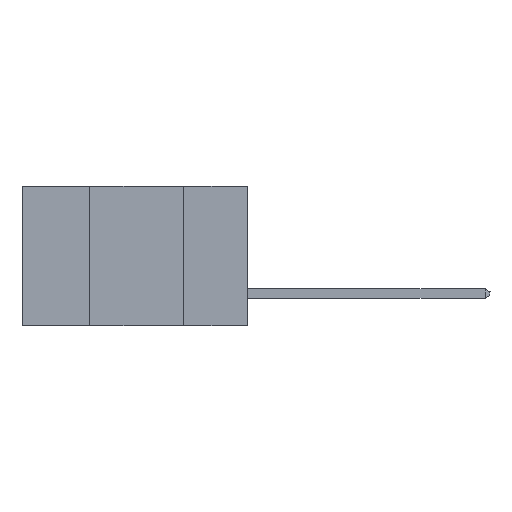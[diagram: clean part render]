
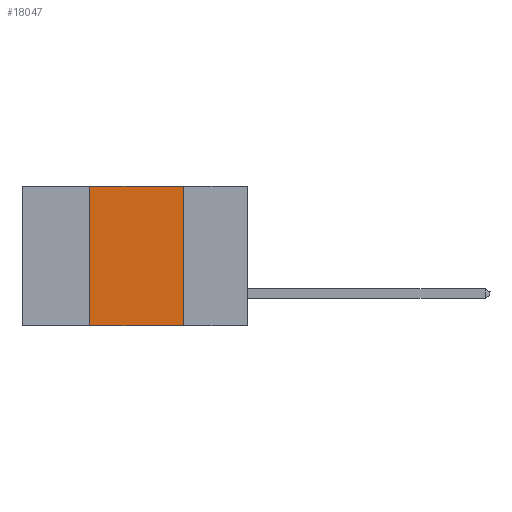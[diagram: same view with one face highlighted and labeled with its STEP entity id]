
A CAD part, left-side view. The second image highlights one B-rep face of the part: STEP entity #18047.
In plain terms, the highlighted planar face has unit normal (-1, 0, 0).
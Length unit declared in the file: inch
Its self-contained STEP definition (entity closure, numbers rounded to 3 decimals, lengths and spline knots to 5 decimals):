
#502 = LINE ( 'NONE', #14498, #7834 ) ;
#1542 = VECTOR ( 'NONE', #5085, 39.37008 ) ;
#1712 = VERTEX_POINT ( 'NONE', #15161 ) ;
#2251 = ORIENTED_EDGE ( 'NONE', *, *, #16528, .F. ) ;
#2305 = DIRECTION ( 'NONE',  ( 0., -1., 0. ) ) ;
#2497 = AXIS2_PLACEMENT_3D ( 'NONE', #5988, #2922, #11907 ) ;
#2922 = DIRECTION ( 'NONE',  ( 1., 0., 0. ) ) ;
#3722 = VERTEX_POINT ( 'NONE', #14908 ) ;
#5085 = DIRECTION ( 'NONE',  ( 0., 0., 1. ) ) ;
#5988 = CARTESIAN_POINT ( 'NONE',  ( 0., 0.6, 0. ) ) ;
#6765 = LINE ( 'NONE', #15477, #15172 ) ;
#7340 = PLANE ( 'NONE',  #2497 ) ;
#7834 = VECTOR ( 'NONE', #17103, 39.37008 ) ;
#8510 = CARTESIAN_POINT ( 'NONE',  ( 0., 0.42, -0.37 ) ) ;
#10065 = ORIENTED_EDGE ( 'NONE', *, *, #11938, .F. ) ;
#10185 = VERTEX_POINT ( 'NONE', #17473 ) ;
#11642 = EDGE_LOOP ( 'NONE', ( #18245, #2251, #10065, #18706 ) ) ;
#11907 = DIRECTION ( 'NONE',  ( 0., 0., -1. ) ) ;
#11938 = EDGE_CURVE ( 'NONE', #16259, #3722, #15846, .T. ) ;
#12761 = CARTESIAN_POINT ( 'NONE',  ( 0., 0.6, -0.37 ) ) ;
#14121 = DIRECTION ( 'NONE',  ( 0., 0., -1. ) ) ;
#14498 = CARTESIAN_POINT ( 'NONE',  ( 0., 0.6, 0. ) ) ;
#14806 = CARTESIAN_POINT ( 'NONE',  ( 0., 0.42, -0.37 ) ) ;
#14908 = CARTESIAN_POINT ( 'NONE',  ( 0., 0.42, 0. ) ) ;
#15161 = CARTESIAN_POINT ( 'NONE',  ( 0., 0.17, 0. ) ) ;
#15172 = VECTOR ( 'NONE', #14121, 39.37008 ) ;
#15477 = CARTESIAN_POINT ( 'NONE',  ( 0., 0.17, -0.37 ) ) ;
#15807 = EDGE_CURVE ( 'NONE', #16259, #10185, #18418, .T. ) ;
#15846 = LINE ( 'NONE', #8510, #1542 ) ;
#16147 = VECTOR ( 'NONE', #2305, 39.37008 ) ;
#16259 = VERTEX_POINT ( 'NONE', #14806 ) ;
#16528 = EDGE_CURVE ( 'NONE', #3722, #1712, #502, .T. ) ;
#17103 = DIRECTION ( 'NONE',  ( 0., -1., 0. ) ) ;
#17473 = CARTESIAN_POINT ( 'NONE',  ( 0., 0.17, -0.37 ) ) ;
#17669 = FACE_OUTER_BOUND ( 'NONE', #11642, .T. ) ;
#17779 = EDGE_CURVE ( 'NONE', #1712, #10185, #6765, .T. ) ;
#18047 = ADVANCED_FACE ( 'NONE', ( #17669 ), #7340, .F. ) ;
#18245 = ORIENTED_EDGE ( 'NONE', *, *, #17779, .F. ) ;
#18418 = LINE ( 'NONE', #12761, #16147 ) ;
#18706 = ORIENTED_EDGE ( 'NONE', *, *, #15807, .T. ) ;
